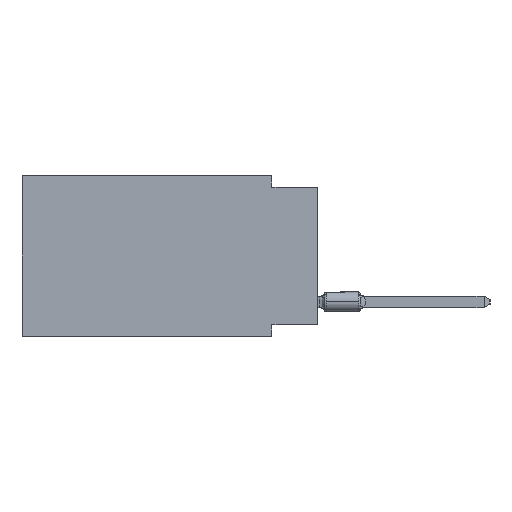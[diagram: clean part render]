
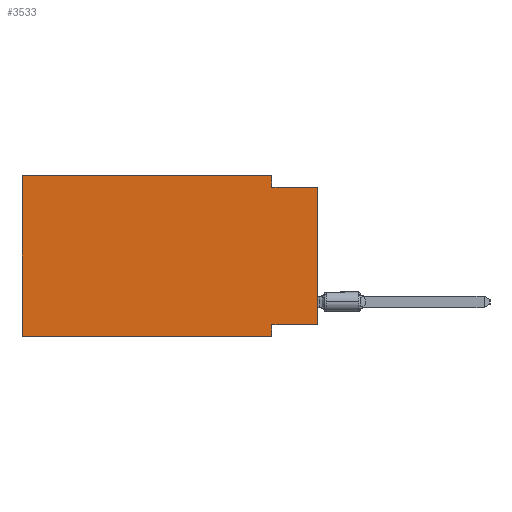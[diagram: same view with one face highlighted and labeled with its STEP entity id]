
A CAD part, left-side view. The second image highlights one B-rep face of the part: STEP entity #3533.
In plain terms, the highlighted planar face has unit normal (-1, 0, 0).
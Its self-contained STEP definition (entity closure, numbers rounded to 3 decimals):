
#964 = DIRECTION ( 'NONE',  ( 0., 0., -1. ) ) ;
#1697 = CARTESIAN_POINT ( 'NONE',  ( 0., 16.383, -8.89 ) ) ;
#2073 = DIRECTION ( 'NONE',  ( 0., 1., 0. ) ) ;
#2475 = DIRECTION ( 'NONE',  ( 0., 0., 1. ) ) ;
#3533 = ADVANCED_FACE ( 'NONE', ( #5877 ), #55793, .F. ) ;
#3902 = DIRECTION ( 'NONE',  ( 0., 0., -1. ) ) ;
#4519 = CARTESIAN_POINT ( 'NONE',  ( 0., 16.383, 0. ) ) ;
#5239 = DIRECTION ( 'NONE',  ( 1., 0., 0. ) ) ;
#5766 = VECTOR ( 'NONE', #2073, 1000. ) ;
#5877 = FACE_OUTER_BOUND ( 'NONE', #60571, .T. ) ;
#7244 = LINE ( 'NONE', #8775, #26795 ) ;
#7353 = CARTESIAN_POINT ( 'NONE',  ( 0., 16.383, -8.89 ) ) ;
#8556 = VECTOR ( 'NONE', #46813, 1000. ) ;
#8650 = VECTOR ( 'NONE', #2475, 1000. ) ;
#8775 = CARTESIAN_POINT ( 'NONE',  ( 0., 16.383, 0. ) ) ;
#9420 = CARTESIAN_POINT ( 'NONE',  ( 0., 2.54, 0. ) ) ;
#10260 = VECTOR ( 'NONE', #964, 1000. ) ;
#10652 = EDGE_CURVE ( 'NONE', #20002, #17222, #64171, .T. ) ;
#12399 = VERTEX_POINT ( 'NONE', #30158 ) ;
#13966 = LINE ( 'NONE', #4519, #27716 ) ;
#14556 = ORIENTED_EDGE ( 'NONE', *, *, #43401, .T. ) ;
#15103 = EDGE_CURVE ( 'NONE', #17634, #59483, #7244, .T. ) ;
#15639 = CARTESIAN_POINT ( 'NONE',  ( 0., 2.54, -8.89 ) ) ;
#16968 = EDGE_CURVE ( 'NONE', #34758, #40388, #20526, .T. ) ;
#17222 = VERTEX_POINT ( 'NONE', #35391 ) ;
#17634 = VERTEX_POINT ( 'NONE', #1697 ) ;
#17827 = VECTOR ( 'NONE', #3902, 1000. ) ;
#18494 = CARTESIAN_POINT ( 'NONE',  ( 0., 2.54, -8.255 ) ) ;
#20002 = VERTEX_POINT ( 'NONE', #39940 ) ;
#20526 = LINE ( 'NONE', #15639, #10260 ) ;
#21002 = CARTESIAN_POINT ( 'NONE',  ( 0., 0., -8.255 ) ) ;
#23122 = ORIENTED_EDGE ( 'NONE', *, *, #16968, .F. ) ;
#24197 = EDGE_CURVE ( 'NONE', #12399, #34758, #51976, .T. ) ;
#24731 = DIRECTION ( 'NONE',  ( 0., -1., 0. ) ) ;
#26795 = VECTOR ( 'NONE', #34199, 1000. ) ;
#27716 = VECTOR ( 'NONE', #24731, 1000. ) ;
#28322 = DIRECTION ( 'NONE',  ( 0., -1., 0. ) ) ;
#29665 = VERTEX_POINT ( 'NONE', #44447 ) ;
#29694 = ORIENTED_EDGE ( 'NONE', *, *, #10652, .F. ) ;
#29963 = EDGE_CURVE ( 'NONE', #59483, #29665, #13966, .T. ) ;
#30158 = CARTESIAN_POINT ( 'NONE',  ( 0., 0., -8.255 ) ) ;
#30352 = CARTESIAN_POINT ( 'NONE',  ( 0., 16.383, 0. ) ) ;
#33411 = CARTESIAN_POINT ( 'NONE',  ( 0., 16.383, 0. ) ) ;
#34199 = DIRECTION ( 'NONE',  ( 0., 0., 1. ) ) ;
#34207 = LINE ( 'NONE', #9420, #17827 ) ;
#34758 = VERTEX_POINT ( 'NONE', #18494 ) ;
#35061 = ORIENTED_EDGE ( 'NONE', *, *, #15103, .F. ) ;
#35391 = CARTESIAN_POINT ( 'NONE',  ( 0., 0., -0.635 ) ) ;
#35789 = ORIENTED_EDGE ( 'NONE', *, *, #42177, .T. ) ;
#39940 = CARTESIAN_POINT ( 'NONE',  ( 0., 2.54, -0.635 ) ) ;
#40388 = VERTEX_POINT ( 'NONE', #40704 ) ;
#40422 = DIRECTION ( 'NONE',  ( 0., 0., -1. ) ) ;
#40704 = CARTESIAN_POINT ( 'NONE',  ( 0., 2.54, -8.89 ) ) ;
#41554 = EDGE_CURVE ( 'NONE', #29665, #20002, #34207, .T. ) ;
#41613 = LINE ( 'NONE', #62494, #8650 ) ;
#42177 = EDGE_CURVE ( 'NONE', #17634, #40388, #56315, .T. ) ;
#43401 = EDGE_CURVE ( 'NONE', #12399, #17222, #41613, .T. ) ;
#44447 = CARTESIAN_POINT ( 'NONE',  ( 0., 2.54, 0. ) ) ;
#46813 = DIRECTION ( 'NONE',  ( 0., -1., 0. ) ) ;
#48521 = CARTESIAN_POINT ( 'NONE',  ( 0., 0., -0.635 ) ) ;
#51877 = AXIS2_PLACEMENT_3D ( 'NONE', #30352, #5239, #40422 ) ;
#51976 = LINE ( 'NONE', #21002, #5766 ) ;
#53694 = ORIENTED_EDGE ( 'NONE', *, *, #29963, .F. ) ;
#54571 = VECTOR ( 'NONE', #28322, 1000. ) ;
#54783 = ORIENTED_EDGE ( 'NONE', *, *, #41554, .F. ) ;
#55403 = ORIENTED_EDGE ( 'NONE', *, *, #24197, .F. ) ;
#55793 = PLANE ( 'NONE',  #51877 ) ;
#56315 = LINE ( 'NONE', #7353, #8556 ) ;
#59483 = VERTEX_POINT ( 'NONE', #33411 ) ;
#60571 = EDGE_LOOP ( 'NONE', ( #14556, #29694, #54783, #53694, #35061, #35789, #23122, #55403 ) ) ;
#62494 = CARTESIAN_POINT ( 'NONE',  ( 0., 0., 0. ) ) ;
#64171 = LINE ( 'NONE', #48521, #54571 ) ;
